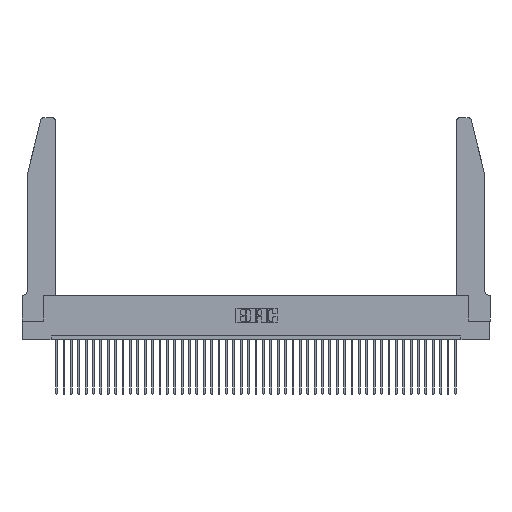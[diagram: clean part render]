
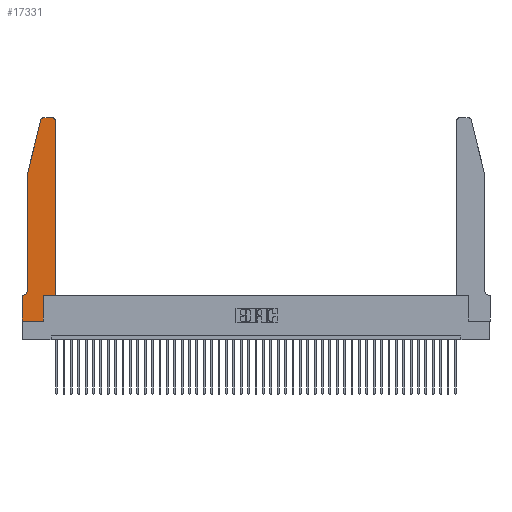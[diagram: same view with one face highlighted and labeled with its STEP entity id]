
A CAD part, top view. The second image highlights one B-rep face of the part: STEP entity #17331.
In plain terms, the highlighted planar face has unit normal (0, 0, 1).
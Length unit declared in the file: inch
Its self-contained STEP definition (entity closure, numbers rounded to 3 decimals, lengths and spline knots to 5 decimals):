
#119 = EDGE_LOOP ( 'NONE', ( #37992, #19308, #23321, #2121, #30303, #27036, #22465, #22416, #16605, #14742, #13403, #14398 ) ) ;
#295 = CARTESIAN_POINT ( 'NONE',  ( 0.0755, 2., 0.37 ) ) ;
#865 = CARTESIAN_POINT ( 'NONE',  ( 0.0755, 0.42, 0.37 ) ) ;
#2121 = ORIENTED_EDGE ( 'NONE', *, *, #36391, .T. ) ;
#2725 = CIRCLE ( 'NONE', #43500, 0.07 ) ;
#2872 = LINE ( 'NONE', #34145, #21547 ) ;
#3005 = LINE ( 'NONE', #34859, #44317 ) ;
#3615 = DIRECTION ( 'NONE',  ( -1., 0., 0. ) ) ;
#3854 = LINE ( 'NONE', #35835, #10807 ) ;
#3918 = DIRECTION ( 'NONE',  ( -0.239, -0.971, 0. ) ) ;
#6612 = AXIS2_PLACEMENT_3D ( 'NONE', #33017, #22673, #26147 ) ;
#6771 = VERTEX_POINT ( 'NONE', #34018 ) ;
#6890 = DIRECTION ( 'NONE',  ( 0., 1., 0. ) ) ;
#8509 = VERTEX_POINT ( 'NONE', #44135 ) ;
#8731 = EDGE_CURVE ( 'NONE', #6771, #8509, #3854, .T. ) ;
#8943 = VECTOR ( 'NONE', #3918, 39.37008 ) ;
#10807 = VECTOR ( 'NONE', #12894, 39.37008 ) ;
#10945 = VECTOR ( 'NONE', #42599, 39.37008 ) ;
#11621 = VECTOR ( 'NONE', #25818, 39.37008 ) ;
#12894 = DIRECTION ( 'NONE',  ( 1., 0., 0. ) ) ;
#12902 = EDGE_CURVE ( 'NONE', #8509, #40926, #27632, .T. ) ;
#13403 = ORIENTED_EDGE ( 'NONE', *, *, #12902, .T. ) ;
#13761 = PLANE ( 'NONE',  #36283 ) ;
#13776 = DIRECTION ( 'NONE',  ( 0., 0., -1. ) ) ;
#13940 = EDGE_CURVE ( 'NONE', #23781, #17531, #15653, .T. ) ;
#14094 = VECTOR ( 'NONE', #35339, 39.37008 ) ;
#14323 = CARTESIAN_POINT ( 'NONE',  ( 0.2865, 0., 0.37 ) ) ;
#14398 = ORIENTED_EDGE ( 'NONE', *, *, #37257, .T. ) ;
#14627 = EDGE_CURVE ( 'NONE', #37669, #23781, #2872, .T. ) ;
#14742 = ORIENTED_EDGE ( 'NONE', *, *, #8731, .T. ) ;
#14806 = LINE ( 'NONE', #28085, #11621 ) ;
#14991 = DIRECTION ( 'NONE',  ( 1., 0., 0. ) ) ;
#15166 = LINE ( 'NONE', #295, #14094 ) ;
#15653 = CIRCLE ( 'NONE', #6612, 0.03 ) ;
#16605 = ORIENTED_EDGE ( 'NONE', *, *, #39859, .T. ) ;
#17069 = CARTESIAN_POINT ( 'NONE',  ( 0., 0.35, 0.37 ) ) ;
#17085 = CARTESIAN_POINT ( 'NONE',  ( 0.0055, 0.42, 0.37 ) ) ;
#17331 = ADVANCED_FACE ( 'NONE', ( #37506 ), #13761, .T. ) ;
#17481 = DIRECTION ( 'NONE',  ( 1., 0., 0. ) ) ;
#17531 = VERTEX_POINT ( 'NONE', #31406 ) ;
#17748 = CIRCLE ( 'NONE', #18022, 0.03 ) ;
#17804 = CARTESIAN_POINT ( 'NONE',  ( 0.0755, 2., 0.37 ) ) ;
#17898 = LINE ( 'NONE', #21773, #23347 ) ;
#18022 = AXIS2_PLACEMENT_3D ( 'NONE', #40161, #21767, #14991 ) ;
#18201 = VERTEX_POINT ( 'NONE', #38759 ) ;
#18479 = DIRECTION ( 'NONE',  ( 0., -1., 0. ) ) ;
#19308 = ORIENTED_EDGE ( 'NONE', *, *, #13940, .T. ) ;
#19837 = VERTEX_POINT ( 'NONE', #25166 ) ;
#21004 = VERTEX_POINT ( 'NONE', #29616 ) ;
#21232 = EDGE_CURVE ( 'NONE', #18201, #30031, #44336, .T. ) ;
#21547 = VECTOR ( 'NONE', #41198, 39.37008 ) ;
#21767 = DIRECTION ( 'NONE',  ( 0., 0., 1. ) ) ;
#21773 = CARTESIAN_POINT ( 'NONE',  ( 0., 0., 0.37 ) ) ;
#22101 = CARTESIAN_POINT ( 'NONE',  ( 0., 0., 0.37 ) ) ;
#22263 = VECTOR ( 'NONE', #18479, 39.37008 ) ;
#22416 = ORIENTED_EDGE ( 'NONE', *, *, #40075, .T. ) ;
#22465 = ORIENTED_EDGE ( 'NONE', *, *, #21232, .T. ) ;
#22673 = DIRECTION ( 'NONE',  ( 0., 0., 1. ) ) ;
#23321 = ORIENTED_EDGE ( 'NONE', *, *, #34729, .T. ) ;
#23347 = VECTOR ( 'NONE', #35002, 39.37008 ) ;
#23781 = VERTEX_POINT ( 'NONE', #41496 ) ;
#24642 = CARTESIAN_POINT ( 'NONE',  ( 0.4205, 2.75, 0.37 ) ) ;
#24708 = VERTEX_POINT ( 'NONE', #14323 ) ;
#25166 = CARTESIAN_POINT ( 'NONE',  ( 0.0755, 2., 0.37 ) ) ;
#25408 = VERTEX_POINT ( 'NONE', #865 ) ;
#25818 = DIRECTION ( 'NONE',  ( -1., 0., 0. ) ) ;
#26147 = DIRECTION ( 'NONE',  ( 1., 0., 0. ) ) ;
#27036 = ORIENTED_EDGE ( 'NONE', *, *, #30011, .T. ) ;
#27437 = DIRECTION ( 'NONE',  ( 0., 0., 1. ) ) ;
#27632 = LINE ( 'NONE', #34805, #10945 ) ;
#28085 = CARTESIAN_POINT ( 'NONE',  ( 0.0755, 0.35, 0.37 ) ) ;
#28763 = LINE ( 'NONE', #17804, #8943 ) ;
#29616 = CARTESIAN_POINT ( 'NONE',  ( 0.0055, 0.35, 0.37 ) ) ;
#30011 = EDGE_CURVE ( 'NONE', #21004, #18201, #14806, .T. ) ;
#30031 = VERTEX_POINT ( 'NONE', #35427 ) ;
#30303 = ORIENTED_EDGE ( 'NONE', *, *, #39269, .T. ) ;
#31406 = CARTESIAN_POINT ( 'NONE',  ( 0.25487, 2.72718, 0.37 ) ) ;
#33017 = CARTESIAN_POINT ( 'NONE',  ( 0.284, 2.72, 0.37 ) ) ;
#34018 = CARTESIAN_POINT ( 'NONE',  ( 0.2865, 0.35, 0.37 ) ) ;
#34145 = CARTESIAN_POINT ( 'NONE',  ( 0.2605, 2.75, 0.37 ) ) ;
#34729 = EDGE_CURVE ( 'NONE', #17531, #19837, #28763, .T. ) ;
#34805 = CARTESIAN_POINT ( 'NONE',  ( 0.4505, 0.35, 0.37 ) ) ;
#34859 = CARTESIAN_POINT ( 'NONE',  ( 0.2865, 0.35, 0.37 ) ) ;
#35002 = DIRECTION ( 'NONE',  ( 1., 0., 0. ) ) ;
#35339 = DIRECTION ( 'NONE',  ( 0., -1., 0. ) ) ;
#35427 = CARTESIAN_POINT ( 'NONE',  ( 0., 0., 0.37 ) ) ;
#35835 = CARTESIAN_POINT ( 'NONE',  ( 0.4505, 0.35, 0.37 ) ) ;
#36283 = AXIS2_PLACEMENT_3D ( 'NONE', #17069, #27437, #17481 ) ;
#36391 = EDGE_CURVE ( 'NONE', #19837, #25408, #15166, .T. ) ;
#37257 = EDGE_CURVE ( 'NONE', #40926, #37669, #17748, .T. ) ;
#37506 = FACE_OUTER_BOUND ( 'NONE', #119, .T. ) ;
#37669 = VERTEX_POINT ( 'NONE', #24642 ) ;
#37992 = ORIENTED_EDGE ( 'NONE', *, *, #14627, .T. ) ;
#38759 = CARTESIAN_POINT ( 'NONE',  ( 0., 0.35, 0.37 ) ) ;
#39269 = EDGE_CURVE ( 'NONE', #25408, #21004, #2725, .T. ) ;
#39859 = EDGE_CURVE ( 'NONE', #24708, #6771, #3005, .T. ) ;
#40075 = EDGE_CURVE ( 'NONE', #30031, #24708, #17898, .T. ) ;
#40161 = CARTESIAN_POINT ( 'NONE',  ( 0.4205, 2.72, 0.37 ) ) ;
#40926 = VERTEX_POINT ( 'NONE', #42754 ) ;
#41198 = DIRECTION ( 'NONE',  ( -1., 0., 0. ) ) ;
#41496 = CARTESIAN_POINT ( 'NONE',  ( 0.284, 2.75, 0.37 ) ) ;
#42599 = DIRECTION ( 'NONE',  ( 0., 1., 0. ) ) ;
#42754 = CARTESIAN_POINT ( 'NONE',  ( 0.4505, 2.72, 0.37 ) ) ;
#43500 = AXIS2_PLACEMENT_3D ( 'NONE', #17085, #13776, #3615 ) ;
#44135 = CARTESIAN_POINT ( 'NONE',  ( 0.4505, 0.35, 0.37 ) ) ;
#44317 = VECTOR ( 'NONE', #6890, 39.37008 ) ;
#44336 = LINE ( 'NONE', #22101, #22263 ) ;
